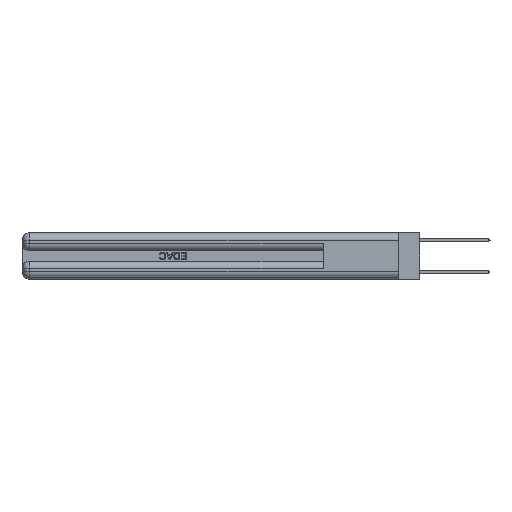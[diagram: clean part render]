
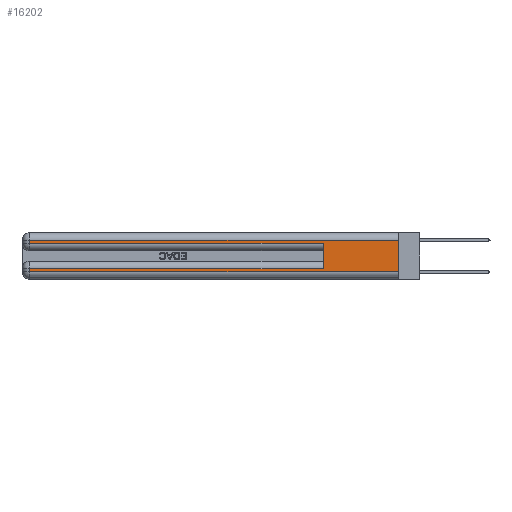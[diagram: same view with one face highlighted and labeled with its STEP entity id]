
A CAD part, left-side view. The second image highlights one B-rep face of the part: STEP entity #16202.
In plain terms, the highlighted planar face has unit normal (-1, 0, 0).
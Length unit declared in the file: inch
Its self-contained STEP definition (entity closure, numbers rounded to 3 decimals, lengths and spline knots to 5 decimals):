
#618 = CARTESIAN_POINT ( 'NONE',  ( 0., 0., 0.06 ) ) ;
#737 = DIRECTION ( 'NONE',  ( 0., -1., 0. ) ) ;
#900 = VECTOR ( 'NONE', #6133, 39.37008 ) ;
#1108 = CARTESIAN_POINT ( 'NONE',  ( 0., 0., 0.37 ) ) ;
#1508 = CARTESIAN_POINT ( 'NONE',  ( 0., 2.94, 0.31 ) ) ;
#1713 = VECTOR ( 'NONE', #7517, 39.37008 ) ;
#2507 = CARTESIAN_POINT ( 'NONE',  ( 0., 0.6, 0.285 ) ) ;
#2886 = CARTESIAN_POINT ( 'NONE',  ( 0., 2.94, 0.37 ) ) ;
#4621 = ORIENTED_EDGE ( 'NONE', *, *, #7469, .T. ) ;
#4674 = LINE ( 'NONE', #13618, #18064 ) ;
#5035 = EDGE_CURVE ( 'NONE', #14934, #23456, #7480, .T. ) ;
#5132 = DIRECTION ( 'NONE',  ( 0., 1., 0. ) ) ;
#5650 = FACE_OUTER_BOUND ( 'NONE', #29088, .T. ) ;
#5996 = CARTESIAN_POINT ( 'NONE',  ( 0., 2.94, 0.285 ) ) ;
#6133 = DIRECTION ( 'NONE',  ( 0., 0., -1. ) ) ;
#6302 = PLANE ( 'NONE',  #31212 ) ;
#6908 = ORIENTED_EDGE ( 'NONE', *, *, #14607, .T. ) ;
#7469 = EDGE_CURVE ( 'NONE', #35224, #36533, #7514, .T. ) ;
#7480 = LINE ( 'NONE', #14983, #22638 ) ;
#7514 = LINE ( 'NONE', #32505, #31087 ) ;
#7517 = DIRECTION ( 'NONE',  ( 0., 1., 0. ) ) ;
#7769 = ORIENTED_EDGE ( 'NONE', *, *, #5035, .T. ) ;
#8041 = VECTOR ( 'NONE', #26831, 39.37008 ) ;
#8518 = LINE ( 'NONE', #17466, #900 ) ;
#8519 = CARTESIAN_POINT ( 'NONE',  ( 0., 0.6, 0.085 ) ) ;
#9155 = ORIENTED_EDGE ( 'NONE', *, *, #28720, .T. ) ;
#9616 = ORIENTED_EDGE ( 'NONE', *, *, #17228, .T. ) ;
#10777 = VERTEX_POINT ( 'NONE', #1508 ) ;
#12026 = DIRECTION ( 'NONE',  ( 0., 0., -1. ) ) ;
#12607 = DIRECTION ( 'NONE',  ( 0., -1., 0. ) ) ;
#12711 = EDGE_CURVE ( 'NONE', #17369, #23456, #24133, .T. ) ;
#13020 = VECTOR ( 'NONE', #19992, 39.37008 ) ;
#13618 = CARTESIAN_POINT ( 'NONE',  ( 0., 0., 0.31 ) ) ;
#14607 = EDGE_CURVE ( 'NONE', #17369, #34163, #25386, .T. ) ;
#14934 = VERTEX_POINT ( 'NONE', #5996 ) ;
#14983 = CARTESIAN_POINT ( 'NONE',  ( 0., 0., 0.285 ) ) ;
#15634 = LINE ( 'NONE', #1108, #8041 ) ;
#16202 = ADVANCED_FACE ( 'NONE', ( #5650 ), #6302, .F. ) ;
#16242 = DIRECTION ( 'NONE',  ( 0., 0., 1. ) ) ;
#17228 = EDGE_CURVE ( 'NONE', #18777, #10777, #4674, .T. ) ;
#17369 = VERTEX_POINT ( 'NONE', #8519 ) ;
#17466 = CARTESIAN_POINT ( 'NONE',  ( 0., 2.94, 0.37 ) ) ;
#18064 = VECTOR ( 'NONE', #5132, 39.37008 ) ;
#18777 = VERTEX_POINT ( 'NONE', #32558 ) ;
#18833 = CARTESIAN_POINT ( 'NONE',  ( 0., 0., 0.085 ) ) ;
#19992 = DIRECTION ( 'NONE',  ( 0., 0., -1. ) ) ;
#22638 = VECTOR ( 'NONE', #737, 39.37008 ) ;
#23289 = CARTESIAN_POINT ( 'NONE',  ( 0., 2.94, 0.06 ) ) ;
#23456 = VERTEX_POINT ( 'NONE', #2507 ) ;
#24133 = LINE ( 'NONE', #36147, #25015 ) ;
#24162 = EDGE_CURVE ( 'NONE', #34163, #35224, #8518, .T. ) ;
#24384 = EDGE_CURVE ( 'NONE', #18777, #36533, #15634, .T. ) ;
#25015 = VECTOR ( 'NONE', #16242, 39.37008 ) ;
#25386 = LINE ( 'NONE', #18833, #1713 ) ;
#26241 = CARTESIAN_POINT ( 'NONE',  ( 0., 0., 0.37 ) ) ;
#26831 = DIRECTION ( 'NONE',  ( 0., 0., -1. ) ) ;
#28362 = ORIENTED_EDGE ( 'NONE', *, *, #24384, .F. ) ;
#28720 = EDGE_CURVE ( 'NONE', #10777, #14934, #34823, .T. ) ;
#29088 = EDGE_LOOP ( 'NONE', ( #28362, #9616, #9155, #7769, #33511, #6908, #35406, #4621 ) ) ;
#29114 = DIRECTION ( 'NONE',  ( 1., 0., 0. ) ) ;
#31087 = VECTOR ( 'NONE', #12607, 39.37008 ) ;
#31212 = AXIS2_PLACEMENT_3D ( 'NONE', #26241, #29114, #12026 ) ;
#32505 = CARTESIAN_POINT ( 'NONE',  ( 0., 0., 0.06 ) ) ;
#32558 = CARTESIAN_POINT ( 'NONE',  ( 0., 0., 0.31 ) ) ;
#33511 = ORIENTED_EDGE ( 'NONE', *, *, #12711, .F. ) ;
#34163 = VERTEX_POINT ( 'NONE', #34932 ) ;
#34823 = LINE ( 'NONE', #2886, #13020 ) ;
#34932 = CARTESIAN_POINT ( 'NONE',  ( 0., 2.94, 0.085 ) ) ;
#35224 = VERTEX_POINT ( 'NONE', #23289 ) ;
#35406 = ORIENTED_EDGE ( 'NONE', *, *, #24162, .T. ) ;
#36147 = CARTESIAN_POINT ( 'NONE',  ( 0., 0.6, 0.145 ) ) ;
#36533 = VERTEX_POINT ( 'NONE', #618 ) ;
